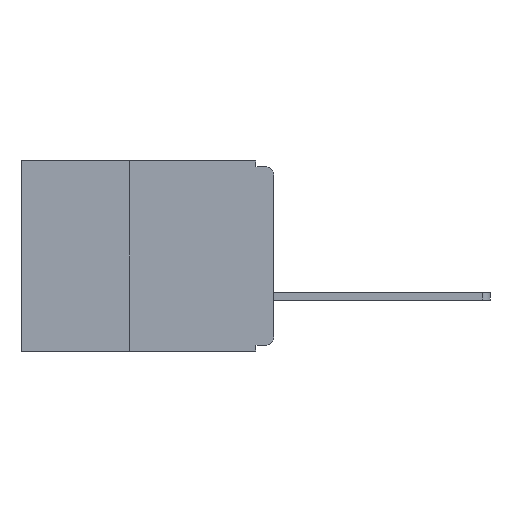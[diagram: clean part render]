
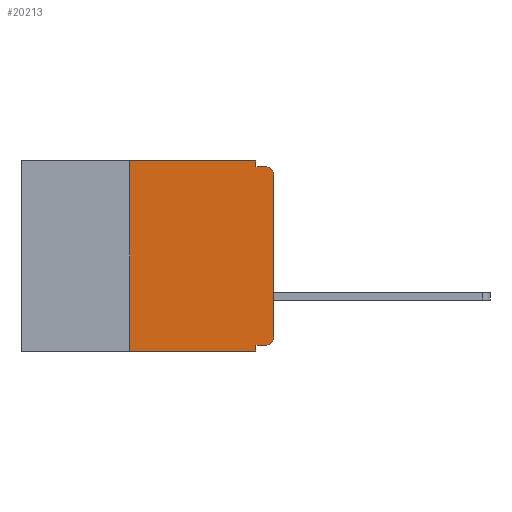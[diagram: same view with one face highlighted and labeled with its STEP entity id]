
A CAD part, left-side view. The second image highlights one B-rep face of the part: STEP entity #20213.
In plain terms, the highlighted planar face has unit normal (-1, 0, 0).
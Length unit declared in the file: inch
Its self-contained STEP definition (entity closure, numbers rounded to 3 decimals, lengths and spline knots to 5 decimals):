
#424 = LINE ( 'NONE', #1728, #6738 ) ;
#584 = CARTESIAN_POINT ( 'NONE',  ( 0., 0.031, 0. ) ) ;
#1728 = CARTESIAN_POINT ( 'NONE',  ( 0., 0.437, 0. ) ) ;
#1743 = CARTESIAN_POINT ( 'NONE',  ( 0., 0., -0.025 ) ) ;
#1932 = EDGE_LOOP ( 'NONE', ( #10403, #2563, #22675, #2392, #8604, #31468, #8384, #3738, #15934, #22451 ) ) ;
#2392 = ORIENTED_EDGE ( 'NONE', *, *, #15285, .F. ) ;
#2563 = ORIENTED_EDGE ( 'NONE', *, *, #3844, .T. ) ;
#2570 = DIRECTION ( 'NONE',  ( -1., 0., 0. ) ) ;
#2628 = LINE ( 'NONE', #4421, #22770 ) ;
#3520 = DIRECTION ( 'NONE',  ( 0., 0., -1. ) ) ;
#3542 = CARTESIAN_POINT ( 'NONE',  ( 0., 0.031, -0.33 ) ) ;
#3738 = ORIENTED_EDGE ( 'NONE', *, *, #15357, .F. ) ;
#3800 = DIRECTION ( 'NONE',  ( -1., 0., 0. ) ) ;
#3844 = EDGE_CURVE ( 'NONE', #17351, #23007, #17186, .T. ) ;
#4145 = CARTESIAN_POINT ( 'NONE',  ( 0., 0.015, -0.025 ) ) ;
#4147 = EDGE_CURVE ( 'NONE', #19036, #23007, #14268, .T. ) ;
#4421 = CARTESIAN_POINT ( 'NONE',  ( 0., 0., -0.32 ) ) ;
#4436 = AXIS2_PLACEMENT_3D ( 'NONE', #4145, #3800, #3520 ) ;
#5257 = PLANE ( 'NONE',  #30137 ) ;
#5275 = EDGE_CURVE ( 'NONE', #11458, #11882, #6492, .T. ) ;
#5955 = VECTOR ( 'NONE', #8861, 39.37008 ) ;
#6492 = LINE ( 'NONE', #23924, #13429 ) ;
#6738 = VECTOR ( 'NONE', #17659, 39.37008 ) ;
#7245 = CARTESIAN_POINT ( 'NONE',  ( 0., 0., 0. ) ) ;
#7292 = VECTOR ( 'NONE', #15351, 39.37008 ) ;
#7926 = DIRECTION ( 'NONE',  ( 0., 0., -1. ) ) ;
#7997 = CARTESIAN_POINT ( 'NONE',  ( 0., 0.031, -0.01 ) ) ;
#8384 = ORIENTED_EDGE ( 'NONE', *, *, #5275, .T. ) ;
#8604 = ORIENTED_EDGE ( 'NONE', *, *, #26166, .F. ) ;
#8861 = DIRECTION ( 'NONE',  ( 0., 0., -1. ) ) ;
#10403 = ORIENTED_EDGE ( 'NONE', *, *, #24435, .T. ) ;
#10412 = CARTESIAN_POINT ( 'NONE',  ( 0., 0.437, 0. ) ) ;
#11458 = VERTEX_POINT ( 'NONE', #27530 ) ;
#11882 = VERTEX_POINT ( 'NONE', #19182 ) ;
#12857 = EDGE_CURVE ( 'NONE', #30435, #14206, #16250, .T. ) ;
#12924 = VERTEX_POINT ( 'NONE', #16052 ) ;
#12925 = LINE ( 'NONE', #3542, #5955 ) ;
#13429 = VECTOR ( 'NONE', #24031, 39.37008 ) ;
#14206 = VERTEX_POINT ( 'NONE', #31406 ) ;
#14268 = LINE ( 'NONE', #20345, #26475 ) ;
#14585 = AXIS2_PLACEMENT_3D ( 'NONE', #18388, #2570, #20962 ) ;
#15113 = DIRECTION ( 'NONE',  ( 0., 0., 1. ) ) ;
#15285 = EDGE_CURVE ( 'NONE', #12924, #19036, #23158, .T. ) ;
#15351 = DIRECTION ( 'NONE',  ( 0., 0., 1. ) ) ;
#15357 = EDGE_CURVE ( 'NONE', #26056, #11882, #12925, .T. ) ;
#15384 = VECTOR ( 'NONE', #29261, 39.37008 ) ;
#15687 = CARTESIAN_POINT ( 'NONE',  ( 0., 0.015, -0.32 ) ) ;
#15934 = ORIENTED_EDGE ( 'NONE', *, *, #30878, .F. ) ;
#16052 = CARTESIAN_POINT ( 'NONE',  ( 0., 0.031, 0. ) ) ;
#16091 = VECTOR ( 'NONE', #15113, 39.37008 ) ;
#16250 = CIRCLE ( 'NONE', #14585, 0.015 ) ;
#16940 = LINE ( 'NONE', #7245, #16091 ) ;
#17186 = CIRCLE ( 'NONE', #4436, 0.015 ) ;
#17202 = CARTESIAN_POINT ( 'NONE',  ( 0., 0.031, -0.32 ) ) ;
#17351 = VERTEX_POINT ( 'NONE', #1743 ) ;
#17659 = DIRECTION ( 'NONE',  ( 0., -1., 0. ) ) ;
#18388 = CARTESIAN_POINT ( 'NONE',  ( 0., 0.015, -0.305 ) ) ;
#19036 = VERTEX_POINT ( 'NONE', #7997 ) ;
#19182 = CARTESIAN_POINT ( 'NONE',  ( 0., 0.031, -0.33 ) ) ;
#19705 = CARTESIAN_POINT ( 'NONE',  ( 0., 0.015, -0.01 ) ) ;
#20117 = DIRECTION ( 'NONE',  ( 0., 1., 0. ) ) ;
#20213 = ADVANCED_FACE ( 'NONE', ( #20898 ), #5257, .F. ) ;
#20345 = CARTESIAN_POINT ( 'NONE',  ( 0., 0., -0.01 ) ) ;
#20382 = DIRECTION ( 'NONE',  ( 0., -1., 0. ) ) ;
#20898 = FACE_OUTER_BOUND ( 'NONE', #1932, .T. ) ;
#20962 = DIRECTION ( 'NONE',  ( 0., 0., -1. ) ) ;
#22451 = ORIENTED_EDGE ( 'NONE', *, *, #12857, .T. ) ;
#22675 = ORIENTED_EDGE ( 'NONE', *, *, #4147, .F. ) ;
#22770 = VECTOR ( 'NONE', #20117, 39.37008 ) ;
#23007 = VERTEX_POINT ( 'NONE', #19705 ) ;
#23158 = LINE ( 'NONE', #584, #15384 ) ;
#23572 = DIRECTION ( 'NONE',  ( 1., 0., 0. ) ) ;
#23924 = CARTESIAN_POINT ( 'NONE',  ( 0., 0.437, -0.33 ) ) ;
#24031 = DIRECTION ( 'NONE',  ( 0., -1., 0. ) ) ;
#24435 = EDGE_CURVE ( 'NONE', #14206, #17351, #16940, .T. ) ;
#26056 = VERTEX_POINT ( 'NONE', #17202 ) ;
#26166 = EDGE_CURVE ( 'NONE', #27928, #12924, #424, .T. ) ;
#26475 = VECTOR ( 'NONE', #20382, 39.37008 ) ;
#27530 = CARTESIAN_POINT ( 'NONE',  ( 0., 0.25, -0.33 ) ) ;
#27928 = VERTEX_POINT ( 'NONE', #29556 ) ;
#27998 = LINE ( 'NONE', #28229, #7292 ) ;
#28229 = CARTESIAN_POINT ( 'NONE',  ( 0., 0.25, -0.33 ) ) ;
#29261 = DIRECTION ( 'NONE',  ( 0., 0., -1. ) ) ;
#29556 = CARTESIAN_POINT ( 'NONE',  ( 0., 0.25, 0. ) ) ;
#30137 = AXIS2_PLACEMENT_3D ( 'NONE', #10412, #23572, #7926 ) ;
#30435 = VERTEX_POINT ( 'NONE', #15687 ) ;
#30878 = EDGE_CURVE ( 'NONE', #30435, #26056, #2628, .T. ) ;
#31406 = CARTESIAN_POINT ( 'NONE',  ( 0., 0., -0.305 ) ) ;
#31468 = ORIENTED_EDGE ( 'NONE', *, *, #33817, .F. ) ;
#33817 = EDGE_CURVE ( 'NONE', #11458, #27928, #27998, .T. ) ;
